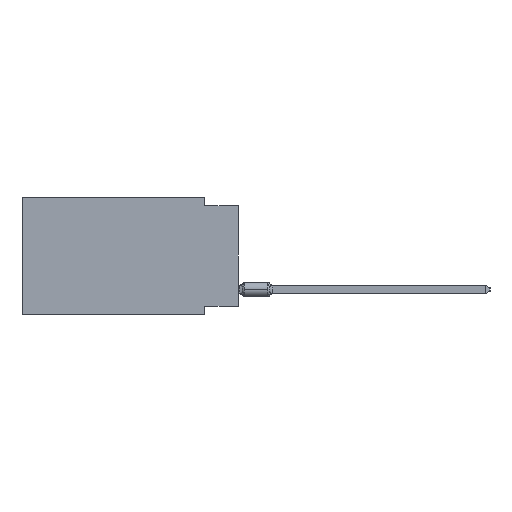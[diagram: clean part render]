
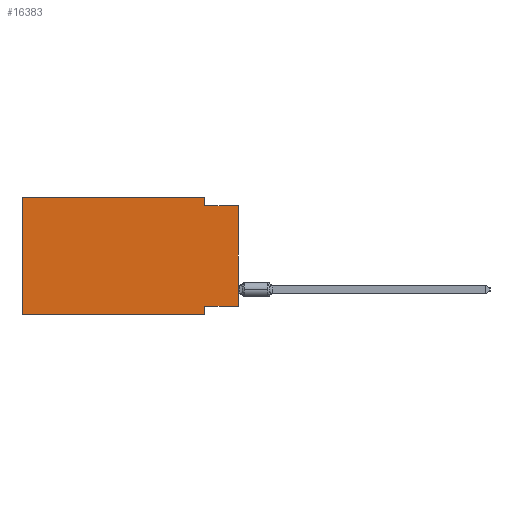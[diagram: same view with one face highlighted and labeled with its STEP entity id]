
A CAD part, left-side view. The second image highlights one B-rep face of the part: STEP entity #16383.
In plain terms, the highlighted planar face has unit normal (-1, 0, 0).
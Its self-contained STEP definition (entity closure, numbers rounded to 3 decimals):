
#792 = DIRECTION ( 'NONE',  ( 0., 1., 0. ) ) ;
#3909 = CARTESIAN_POINT ( 'NONE',  ( 0., 2.54, -0.635 ) ) ;
#3994 = EDGE_CURVE ( 'NONE', #87143, #41160, #83934, .T. ) ;
#5831 = CARTESIAN_POINT ( 'NONE',  ( 0., 16.383, 0. ) ) ;
#9737 = ORIENTED_EDGE ( 'NONE', *, *, #3994, .F. ) ;
#11998 = ORIENTED_EDGE ( 'NONE', *, *, #66830, .F. ) ;
#12486 = VECTOR ( 'NONE', #45735, 1000. ) ;
#14074 = VERTEX_POINT ( 'NONE', #31838 ) ;
#14962 = DIRECTION ( 'NONE',  ( 0., -1., 0. ) ) ;
#16131 = DIRECTION ( 'NONE',  ( 0., 0., -1. ) ) ;
#16383 = ADVANCED_FACE ( 'NONE', ( #38467 ), #37548, .F. ) ;
#19766 = EDGE_LOOP ( 'NONE', ( #33119, #9737, #86479, #47513, #11998, #33642, #20535, #55120 ) ) ;
#20535 = ORIENTED_EDGE ( 'NONE', *, *, #60752, .F. ) ;
#20983 = DIRECTION ( 'NONE',  ( 0., 0., -1. ) ) ;
#22156 = CARTESIAN_POINT ( 'NONE',  ( 0., 0., -8.255 ) ) ;
#22917 = VERTEX_POINT ( 'NONE', #22156 ) ;
#24703 = VECTOR ( 'NONE', #20983, 1000. ) ;
#25402 = LINE ( 'NONE', #25864, #75462 ) ;
#25730 = DIRECTION ( 'NONE',  ( 0., -1., 0. ) ) ;
#25864 = CARTESIAN_POINT ( 'NONE',  ( 0., 2.54, 0. ) ) ;
#26202 = CARTESIAN_POINT ( 'NONE',  ( 0., 2.54, -8.255 ) ) ;
#30936 = DIRECTION ( 'NONE',  ( 0., -1., 0. ) ) ;
#31838 = CARTESIAN_POINT ( 'NONE',  ( 0., 16.383, -8.89 ) ) ;
#33119 = ORIENTED_EDGE ( 'NONE', *, *, #82410, .T. ) ;
#33642 = ORIENTED_EDGE ( 'NONE', *, *, #74123, .T. ) ;
#34207 = DIRECTION ( 'NONE',  ( 0., 0., 1. ) ) ;
#34784 = LINE ( 'NONE', #49692, #51941 ) ;
#36291 = CARTESIAN_POINT ( 'NONE',  ( 0., 2.54, -8.89 ) ) ;
#37548 = PLANE ( 'NONE',  #67977 ) ;
#37817 = CARTESIAN_POINT ( 'NONE',  ( 0., 0., 0. ) ) ;
#37929 = LINE ( 'NONE', #66334, #81565 ) ;
#38467 = FACE_OUTER_BOUND ( 'NONE', #19766, .T. ) ;
#41160 = VERTEX_POINT ( 'NONE', #67864 ) ;
#42450 = CARTESIAN_POINT ( 'NONE',  ( 0., 16.383, -8.89 ) ) ;
#45341 = CARTESIAN_POINT ( 'NONE',  ( 0., 2.54, 0. ) ) ;
#45735 = DIRECTION ( 'NONE',  ( 0., 0., 1. ) ) ;
#47513 = ORIENTED_EDGE ( 'NONE', *, *, #89028, .F. ) ;
#49692 = CARTESIAN_POINT ( 'NONE',  ( 0., 0., -8.255 ) ) ;
#51941 = VECTOR ( 'NONE', #792, 1000. ) ;
#51981 = CARTESIAN_POINT ( 'NONE',  ( 0., 16.383, 0. ) ) ;
#54093 = VECTOR ( 'NONE', #14962, 1000. ) ;
#54959 = VERTEX_POINT ( 'NONE', #45341 ) ;
#55120 = ORIENTED_EDGE ( 'NONE', *, *, #64634, .F. ) ;
#59897 = DIRECTION ( 'NONE',  ( 1., 0., 0. ) ) ;
#60752 = EDGE_CURVE ( 'NONE', #84355, #77358, #65140, .T. ) ;
#62217 = EDGE_CURVE ( 'NONE', #54959, #87143, #25402, .T. ) ;
#64634 = EDGE_CURVE ( 'NONE', #22917, #84355, #34784, .T. ) ;
#65140 = LINE ( 'NONE', #36291, #24703 ) ;
#66334 = CARTESIAN_POINT ( 'NONE',  ( 0., 16.383, 0. ) ) ;
#66830 = EDGE_CURVE ( 'NONE', #14074, #91330, #90573, .T. ) ;
#67864 = CARTESIAN_POINT ( 'NONE',  ( 0., 0., -0.635 ) ) ;
#67977 = AXIS2_PLACEMENT_3D ( 'NONE', #51981, #59897, #16131 ) ;
#71771 = LINE ( 'NONE', #42450, #54093 ) ;
#74123 = EDGE_CURVE ( 'NONE', #14074, #77358, #71771, .T. ) ;
#75462 = VECTOR ( 'NONE', #84068, 1000. ) ;
#77358 = VERTEX_POINT ( 'NONE', #89517 ) ;
#78418 = LINE ( 'NONE', #37817, #12486 ) ;
#79900 = CARTESIAN_POINT ( 'NONE',  ( 0., 16.383, 0. ) ) ;
#81565 = VECTOR ( 'NONE', #30936, 1000. ) ;
#82088 = CARTESIAN_POINT ( 'NONE',  ( 0., 0., -0.635 ) ) ;
#82410 = EDGE_CURVE ( 'NONE', #22917, #41160, #78418, .T. ) ;
#83934 = LINE ( 'NONE', #82088, #85869 ) ;
#84068 = DIRECTION ( 'NONE',  ( 0., 0., -1. ) ) ;
#84355 = VERTEX_POINT ( 'NONE', #26202 ) ;
#85869 = VECTOR ( 'NONE', #25730, 1000. ) ;
#86479 = ORIENTED_EDGE ( 'NONE', *, *, #62217, .F. ) ;
#87143 = VERTEX_POINT ( 'NONE', #3909 ) ;
#89028 = EDGE_CURVE ( 'NONE', #91330, #54959, #37929, .T. ) ;
#89178 = VECTOR ( 'NONE', #34207, 1000. ) ;
#89517 = CARTESIAN_POINT ( 'NONE',  ( 0., 2.54, -8.89 ) ) ;
#90573 = LINE ( 'NONE', #5831, #89178 ) ;
#91330 = VERTEX_POINT ( 'NONE', #79900 ) ;
